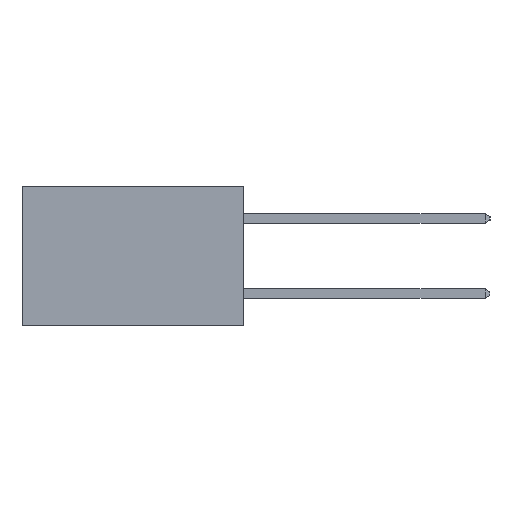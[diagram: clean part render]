
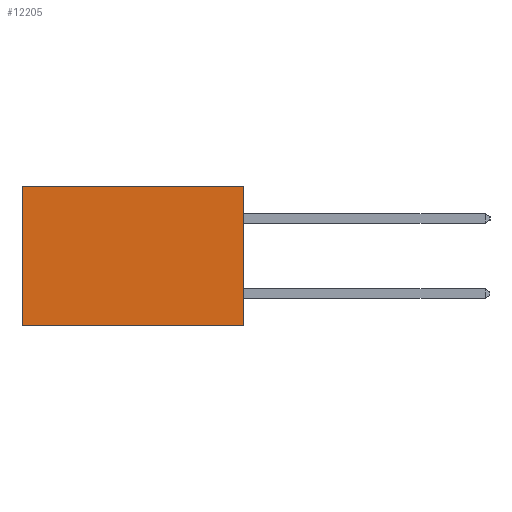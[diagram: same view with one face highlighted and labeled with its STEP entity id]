
A CAD part, left-side view. The second image highlights one B-rep face of the part: STEP entity #12205.
In plain terms, the highlighted planar face has unit normal (-1, 0, 0).
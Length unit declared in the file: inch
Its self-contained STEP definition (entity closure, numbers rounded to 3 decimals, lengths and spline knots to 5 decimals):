
#79 = EDGE_CURVE ( 'NONE', #15846, #18185, #4494, .T. ) ;
#161 = ORIENTED_EDGE ( 'NONE', *, *, #10668, .T. ) ;
#211 = CARTESIAN_POINT ( 'NONE',  ( 0.277, 0.59, -0.37 ) ) ;
#1237 = EDGE_CURVE ( 'NONE', #18185, #1499, #14076, .T. ) ;
#1268 = CARTESIAN_POINT ( 'NONE',  ( 0.277, 0., 0. ) ) ;
#1499 = VERTEX_POINT ( 'NONE', #9287 ) ;
#1607 = CARTESIAN_POINT ( 'NONE',  ( 0.277, 0., -0.37 ) ) ;
#2662 = PLANE ( 'NONE',  #6783 ) ;
#2921 = ORIENTED_EDGE ( 'NONE', *, *, #13787, .T. ) ;
#4383 = VERTEX_POINT ( 'NONE', #8648 ) ;
#4466 = DIRECTION ( 'NONE',  ( 0., 1., 0. ) ) ;
#4494 = LINE ( 'NONE', #21096, #17005 ) ;
#4816 = ORIENTED_EDGE ( 'NONE', *, *, #79, .F. ) ;
#6204 = FACE_OUTER_BOUND ( 'NONE', #11403, .T. ) ;
#6257 = DIRECTION ( 'NONE',  ( 1., 0., 0. ) ) ;
#6281 = LINE ( 'NONE', #211, #11352 ) ;
#6783 = AXIS2_PLACEMENT_3D ( 'NONE', #21271, #6257, #18059 ) ;
#8569 = LINE ( 'NONE', #19871, #21865 ) ;
#8648 = CARTESIAN_POINT ( 'NONE',  ( 0.277, 0.59, 0. ) ) ;
#9287 = CARTESIAN_POINT ( 'NONE',  ( 0.277, 0.59, -0.37 ) ) ;
#9871 = DIRECTION ( 'NONE',  ( 0., 1., 0. ) ) ;
#10602 = CARTESIAN_POINT ( 'NONE',  ( 0.277, 0., -0.37 ) ) ;
#10668 = EDGE_CURVE ( 'NONE', #4383, #1499, #6281, .T. ) ;
#11352 = VECTOR ( 'NONE', #12376, 39.37008 ) ;
#11403 = EDGE_LOOP ( 'NONE', ( #161, #20884, #4816, #2921 ) ) ;
#12205 = ADVANCED_FACE ( 'NONE', ( #6204 ), #2662, .F. ) ;
#12376 = DIRECTION ( 'NONE',  ( 0., 0., -1. ) ) ;
#13787 = EDGE_CURVE ( 'NONE', #15846, #4383, #8569, .T. ) ;
#14076 = LINE ( 'NONE', #1607, #18475 ) ;
#15846 = VERTEX_POINT ( 'NONE', #1268 ) ;
#15868 = DIRECTION ( 'NONE',  ( 0., 0., -1. ) ) ;
#17005 = VECTOR ( 'NONE', #15868, 39.37008 ) ;
#18059 = DIRECTION ( 'NONE',  ( 0., 0., -1. ) ) ;
#18185 = VERTEX_POINT ( 'NONE', #10602 ) ;
#18475 = VECTOR ( 'NONE', #4466, 39.37008 ) ;
#19871 = CARTESIAN_POINT ( 'NONE',  ( 0.277, 0., 0. ) ) ;
#20884 = ORIENTED_EDGE ( 'NONE', *, *, #1237, .F. ) ;
#21096 = CARTESIAN_POINT ( 'NONE',  ( 0.277, 0., -0.37 ) ) ;
#21271 = CARTESIAN_POINT ( 'NONE',  ( 0.277, 0., -0.37 ) ) ;
#21865 = VECTOR ( 'NONE', #9871, 39.37008 ) ;
